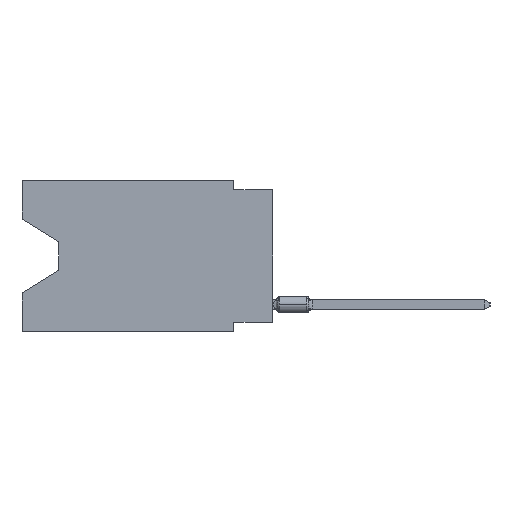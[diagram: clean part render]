
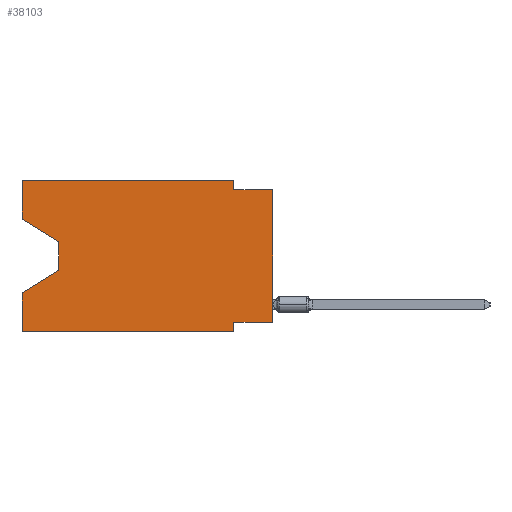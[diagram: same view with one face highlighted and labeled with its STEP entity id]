
A CAD part, left-side view. The second image highlights one B-rep face of the part: STEP entity #38103.
In plain terms, the highlighted planar face has unit normal (-1, 0, 0).
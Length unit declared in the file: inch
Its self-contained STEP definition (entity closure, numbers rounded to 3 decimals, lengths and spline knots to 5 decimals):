
#233 = EDGE_CURVE ( 'NONE', #8531, #40688, #2144, .T. ) ;
#547 = LINE ( 'NONE', #26945, #5471 ) ;
#641 = LINE ( 'NONE', #44189, #6643 ) ;
#1076 = DIRECTION ( 'NONE',  ( 0., 0., 1. ) ) ;
#1555 = CARTESIAN_POINT ( 'NONE',  ( 0., 0.645, 0. ) ) ;
#2144 = LINE ( 'NONE', #45693, #39772 ) ;
#2458 = CARTESIAN_POINT ( 'NONE',  ( 0., 0.645, 0. ) ) ;
#2615 = DIRECTION ( 'NONE',  ( 0., 0.855, -0.519 ) ) ;
#3308 = LINE ( 'NONE', #21108, #28368 ) ;
#4664 = DIRECTION ( 'NONE',  ( 0., 0., 1. ) ) ;
#4893 = CARTESIAN_POINT ( 'NONE',  ( 0., 0.645, -0.39 ) ) ;
#5471 = VECTOR ( 'NONE', #44560, 39.37008 ) ;
#5927 = DIRECTION ( 'NONE',  ( 0., -1., 0. ) ) ;
#5936 = EDGE_CURVE ( 'NONE', #33954, #8531, #8822, .T. ) ;
#6643 = VECTOR ( 'NONE', #11574, 39.37008 ) ;
#6804 = CARTESIAN_POINT ( 'NONE',  ( 0., 0.645, -0.10025 ) ) ;
#7083 = EDGE_LOOP ( 'NONE', ( #38293, #37178, #28068, #25269, #12676, #37133, #8547, #29633, #39160, #19773, #20500, #7476 ) ) ;
#7476 = ORIENTED_EDGE ( 'NONE', *, *, #17158, .F. ) ;
#7742 = CARTESIAN_POINT ( 'NONE',  ( 0., 0.1, 0. ) ) ;
#8531 = VERTEX_POINT ( 'NONE', #39714 ) ;
#8547 = ORIENTED_EDGE ( 'NONE', *, *, #40012, .F. ) ;
#8596 = DIRECTION ( 'NONE',  ( 0., 0., -1. ) ) ;
#8822 = LINE ( 'NONE', #11900, #40171 ) ;
#8903 = VERTEX_POINT ( 'NONE', #10614 ) ;
#10614 = CARTESIAN_POINT ( 'NONE',  ( 0., 0.1, -0.365 ) ) ;
#10626 = AXIS2_PLACEMENT_3D ( 'NONE', #29862, #37720, #37487 ) ;
#11261 = VECTOR ( 'NONE', #4664, 39.37008 ) ;
#11460 = VERTEX_POINT ( 'NONE', #26372 ) ;
#11574 = DIRECTION ( 'NONE',  ( 0., 0., -1. ) ) ;
#11854 = VERTEX_POINT ( 'NONE', #2458 ) ;
#11900 = CARTESIAN_POINT ( 'NONE',  ( 0., 0.55, -0.158 ) ) ;
#12676 = ORIENTED_EDGE ( 'NONE', *, *, #43815, .T. ) ;
#14293 = VERTEX_POINT ( 'NONE', #6804 ) ;
#15598 = CARTESIAN_POINT ( 'NONE',  ( 0., 0.55, -0.158 ) ) ;
#16075 = EDGE_CURVE ( 'NONE', #17125, #46538, #33205, .T. ) ;
#16575 = VECTOR ( 'NONE', #44415, 39.37008 ) ;
#16822 = DIRECTION ( 'NONE',  ( 0., -1., 0. ) ) ;
#17089 = EDGE_CURVE ( 'NONE', #8903, #37453, #41829, .T. ) ;
#17125 = VERTEX_POINT ( 'NONE', #32984 ) ;
#17158 = EDGE_CURVE ( 'NONE', #14293, #11854, #43696, .T. ) ;
#18643 = FACE_OUTER_BOUND ( 'NONE', #7083, .T. ) ;
#18819 = CARTESIAN_POINT ( 'NONE',  ( 0., 0.645, -0.10025 ) ) ;
#19361 = CARTESIAN_POINT ( 'NONE',  ( 0., 0., 0. ) ) ;
#19773 = ORIENTED_EDGE ( 'NONE', *, *, #41217, .F. ) ;
#20126 = CARTESIAN_POINT ( 'NONE',  ( 0., 0.1, -0.39 ) ) ;
#20500 = ORIENTED_EDGE ( 'NONE', *, *, #25386, .F. ) ;
#21108 = CARTESIAN_POINT ( 'NONE',  ( 0., 0.645, 0. ) ) ;
#21200 = VECTOR ( 'NONE', #28948, 39.37008 ) ;
#21380 = EDGE_CURVE ( 'NONE', #14293, #33954, #22406, .T. ) ;
#22406 = LINE ( 'NONE', #18819, #31271 ) ;
#22939 = PLANE ( 'NONE',  #10626 ) ;
#25269 = ORIENTED_EDGE ( 'NONE', *, *, #41660, .F. ) ;
#25386 = EDGE_CURVE ( 'NONE', #11854, #38145, #3308, .T. ) ;
#26372 = CARTESIAN_POINT ( 'NONE',  ( 0., 0.1, -0.025 ) ) ;
#26521 = EDGE_CURVE ( 'NONE', #11460, #46538, #547, .T. ) ;
#26945 = CARTESIAN_POINT ( 'NONE',  ( 0., 0., -0.025 ) ) ;
#28068 = ORIENTED_EDGE ( 'NONE', *, *, #233, .T. ) ;
#28368 = VECTOR ( 'NONE', #5927, 39.37008 ) ;
#28728 = LINE ( 'NONE', #43263, #16575 ) ;
#28948 = DIRECTION ( 'NONE',  ( 0., 0., 1. ) ) ;
#29633 = ORIENTED_EDGE ( 'NONE', *, *, #16075, .T. ) ;
#29862 = CARTESIAN_POINT ( 'NONE',  ( 0., 0.645, 0. ) ) ;
#31271 = VECTOR ( 'NONE', #33378, 39.37008 ) ;
#32984 = CARTESIAN_POINT ( 'NONE',  ( 0., 0., -0.365 ) ) ;
#33205 = LINE ( 'NONE', #19361, #11261 ) ;
#33378 = DIRECTION ( 'NONE',  ( 0., -0.855, -0.519 ) ) ;
#33901 = LINE ( 'NONE', #1555, #38592 ) ;
#33954 = VERTEX_POINT ( 'NONE', #15598 ) ;
#34933 = LINE ( 'NONE', #43888, #39525 ) ;
#37133 = ORIENTED_EDGE ( 'NONE', *, *, #17089, .F. ) ;
#37178 = ORIENTED_EDGE ( 'NONE', *, *, #5936, .T. ) ;
#37453 = VERTEX_POINT ( 'NONE', #42157 ) ;
#37487 = DIRECTION ( 'NONE',  ( 0., 0., -1. ) ) ;
#37720 = DIRECTION ( 'NONE',  ( 1., 0., 0. ) ) ;
#38103 = ADVANCED_FACE ( 'NONE', ( #18643 ), #22939, .F. ) ;
#38128 = VERTEX_POINT ( 'NONE', #4893 ) ;
#38145 = VERTEX_POINT ( 'NONE', #7742 ) ;
#38293 = ORIENTED_EDGE ( 'NONE', *, *, #21380, .T. ) ;
#38592 = VECTOR ( 'NONE', #1076, 39.37008 ) ;
#39160 = ORIENTED_EDGE ( 'NONE', *, *, #26521, .F. ) ;
#39525 = VECTOR ( 'NONE', #16822, 39.37008 ) ;
#39714 = CARTESIAN_POINT ( 'NONE',  ( 0., 0.55, -0.232 ) ) ;
#39772 = VECTOR ( 'NONE', #2615, 39.37008 ) ;
#40012 = EDGE_CURVE ( 'NONE', #17125, #8903, #28728, .T. ) ;
#40171 = VECTOR ( 'NONE', #8596, 39.37008 ) ;
#40688 = VERTEX_POINT ( 'NONE', #41502 ) ;
#41217 = EDGE_CURVE ( 'NONE', #38145, #11460, #641, .T. ) ;
#41218 = CARTESIAN_POINT ( 'NONE',  ( 0., 0., -0.025 ) ) ;
#41502 = CARTESIAN_POINT ( 'NONE',  ( 0., 0.645, -0.28975 ) ) ;
#41660 = EDGE_CURVE ( 'NONE', #38128, #40688, #33901, .T. ) ;
#41829 = LINE ( 'NONE', #20126, #45562 ) ;
#42157 = CARTESIAN_POINT ( 'NONE',  ( 0., 0.1, -0.39 ) ) ;
#43263 = CARTESIAN_POINT ( 'NONE',  ( 0., 0., -0.365 ) ) ;
#43696 = LINE ( 'NONE', #47025, #21200 ) ;
#43815 = EDGE_CURVE ( 'NONE', #38128, #37453, #34933, .T. ) ;
#43888 = CARTESIAN_POINT ( 'NONE',  ( 0., 0.645, -0.39 ) ) ;
#44189 = CARTESIAN_POINT ( 'NONE',  ( 0., 0.1, 0. ) ) ;
#44415 = DIRECTION ( 'NONE',  ( 0., 1., 0. ) ) ;
#44560 = DIRECTION ( 'NONE',  ( 0., -1., 0. ) ) ;
#45562 = VECTOR ( 'NONE', #45629, 39.37008 ) ;
#45629 = DIRECTION ( 'NONE',  ( 0., 0., -1. ) ) ;
#45693 = CARTESIAN_POINT ( 'NONE',  ( 0., 0.55, -0.232 ) ) ;
#46538 = VERTEX_POINT ( 'NONE', #41218 ) ;
#47025 = CARTESIAN_POINT ( 'NONE',  ( 0., 0.645, 0. ) ) ;
